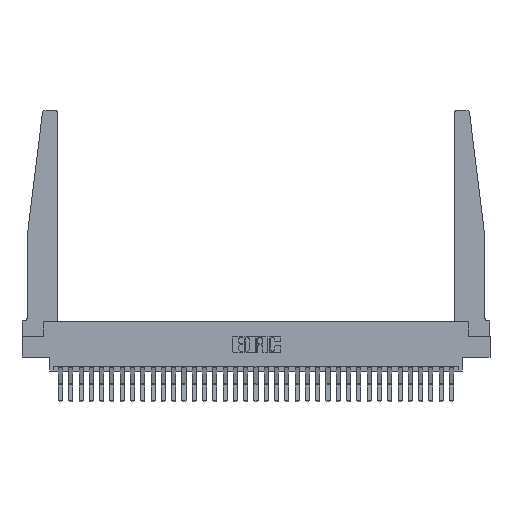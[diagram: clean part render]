
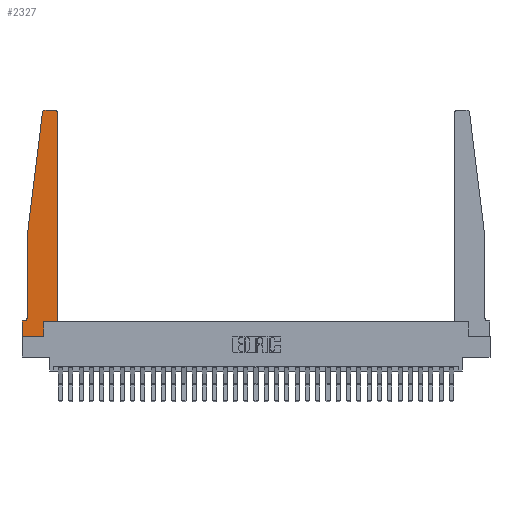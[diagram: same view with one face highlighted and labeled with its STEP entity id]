
A CAD part, top view. The second image highlights one B-rep face of the part: STEP entity #2327.
In plain terms, the highlighted planar face has unit normal (0, 0, 1).
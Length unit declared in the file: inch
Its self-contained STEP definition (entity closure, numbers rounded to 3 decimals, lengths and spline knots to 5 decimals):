
#421 = DIRECTION ( 'NONE',  ( -1., 0., 0. ) ) ;
#681 = VERTEX_POINT ( 'NONE', #3958 ) ;
#983 = VERTEX_POINT ( 'NONE', #4338 ) ;
#1861 = ORIENTED_EDGE ( 'NONE', *, *, #19803, .T. ) ;
#2134 = DIRECTION ( 'NONE',  ( 1., 0., 0. ) ) ;
#2315 = LINE ( 'NONE', #6900, #6386 ) ;
#2326 = ORIENTED_EDGE ( 'NONE', *, *, #6308, .T. ) ;
#2327 = ADVANCED_FACE ( 'NONE', ( #4654 ), #8937, .T. ) ;
#2483 = ORIENTED_EDGE ( 'NONE', *, *, #20605, .T. ) ;
#2792 = VECTOR ( 'NONE', #24482, 39.37008 ) ;
#2905 = VERTEX_POINT ( 'NONE', #14592 ) ;
#3089 = LINE ( 'NONE', #12745, #2792 ) ;
#3877 = VERTEX_POINT ( 'NONE', #20124 ) ;
#3941 = CARTESIAN_POINT ( 'NONE',  ( 0.395, 2.72, 0.37 ) ) ;
#3958 = CARTESIAN_POINT ( 'NONE',  ( 0.395, 2.75, 0.37 ) ) ;
#4250 = CARTESIAN_POINT ( 'NONE',  ( 0.065, 1.25, 0.37 ) ) ;
#4338 = CARTESIAN_POINT ( 'NONE',  ( 0.2605, 0.18, 0.37 ) ) ;
#4415 = ORIENTED_EDGE ( 'NONE', *, *, #16764, .T. ) ;
#4654 = FACE_OUTER_BOUND ( 'NONE', #31258, .T. ) ;
#4717 = VERTEX_POINT ( 'NONE', #27484 ) ;
#4791 = CIRCLE ( 'NONE', #18977, 0.03 ) ;
#5260 = VECTOR ( 'NONE', #11361, 39.37008 ) ;
#5397 = ORIENTED_EDGE ( 'NONE', *, *, #14882, .T. ) ;
#6088 = ORIENTED_EDGE ( 'NONE', *, *, #12064, .T. ) ;
#6089 = VECTOR ( 'NONE', #6155, 39.37008 ) ;
#6155 = DIRECTION ( 'NONE',  ( 0., 1., 0. ) ) ;
#6308 = EDGE_CURVE ( 'NONE', #19038, #23447, #10160, .T. ) ;
#6386 = VECTOR ( 'NONE', #28279, 39.37008 ) ;
#6743 = VERTEX_POINT ( 'NONE', #19764 ) ;
#6900 = CARTESIAN_POINT ( 'NONE',  ( 0.25, 2.75, 0.37 ) ) ;
#7389 = LINE ( 'NONE', #12448, #30969 ) ;
#7442 = CARTESIAN_POINT ( 'NONE',  ( 0.425, 0.18, 0.37 ) ) ;
#7578 = CARTESIAN_POINT ( 'NONE',  ( 0.015, 0.2375, 0.37 ) ) ;
#7744 = DIRECTION ( 'NONE',  ( 1., 0., 0. ) ) ;
#8322 = EDGE_CURVE ( 'NONE', #2905, #19038, #23894, .T. ) ;
#8937 = PLANE ( 'NONE',  #20198 ) ;
#9259 = CARTESIAN_POINT ( 'NONE',  ( 0., 0.1875, 0.37 ) ) ;
#9365 = EDGE_CURVE ( 'NONE', #21525, #983, #3089, .T. ) ;
#9889 = ORIENTED_EDGE ( 'NONE', *, *, #14548, .T. ) ;
#10160 = LINE ( 'NONE', #25352, #28946 ) ;
#11048 = LINE ( 'NONE', #18055, #6089 ) ;
#11361 = DIRECTION ( 'NONE',  ( -0.122, -0.992, 0. ) ) ;
#12064 = EDGE_CURVE ( 'NONE', #4717, #21525, #22014, .T. ) ;
#12083 = CARTESIAN_POINT ( 'NONE',  ( 0.065, 1.25, 0.37 ) ) ;
#12448 = CARTESIAN_POINT ( 'NONE',  ( 0.065, 0.1875, 0.37 ) ) ;
#12745 = CARTESIAN_POINT ( 'NONE',  ( 0.2605, 0.18, 0.37 ) ) ;
#13097 = VECTOR ( 'NONE', #20779, 39.37008 ) ;
#13177 = ORIENTED_EDGE ( 'NONE', *, *, #8322, .T. ) ;
#13376 = CIRCLE ( 'NONE', #22991, 0.03 ) ;
#13601 = DIRECTION ( 'NONE',  ( 0., 0., 1. ) ) ;
#14065 = VERTEX_POINT ( 'NONE', #17497 ) ;
#14548 = EDGE_CURVE ( 'NONE', #21659, #681, #13376, .T. ) ;
#14565 = CARTESIAN_POINT ( 'NONE',  ( 0.27653, 2.72, 0.37 ) ) ;
#14592 = CARTESIAN_POINT ( 'NONE',  ( 0.24675, 2.72367, 0.37 ) ) ;
#14882 = EDGE_CURVE ( 'NONE', #14065, #2905, #4791, .T. ) ;
#15247 = VERTEX_POINT ( 'NONE', #19279 ) ;
#15493 = CARTESIAN_POINT ( 'NONE',  ( 0.2605, 0., 0.37 ) ) ;
#15841 = DIRECTION ( 'NONE',  ( 1., 0., 0. ) ) ;
#16133 = EDGE_CURVE ( 'NONE', #983, #6743, #29144, .T. ) ;
#16400 = VECTOR ( 'NONE', #29135, 39.37008 ) ;
#16764 = EDGE_CURVE ( 'NONE', #681, #14065, #2315, .T. ) ;
#17497 = CARTESIAN_POINT ( 'NONE',  ( 0.27653, 2.75, 0.37 ) ) ;
#17952 = EDGE_CURVE ( 'NONE', #3877, #4717, #18243, .T. ) ;
#18055 = CARTESIAN_POINT ( 'NONE',  ( 0.425, 0.18, 0.37 ) ) ;
#18243 = LINE ( 'NONE', #27896, #13097 ) ;
#18793 = CIRCLE ( 'NONE', #21830, 0.05 ) ;
#18930 = DIRECTION ( 'NONE',  ( 0., 0., 1. ) ) ;
#18977 = AXIS2_PLACEMENT_3D ( 'NONE', #14565, #29446, #7744 ) ;
#19038 = VERTEX_POINT ( 'NONE', #12083 ) ;
#19279 = CARTESIAN_POINT ( 'NONE',  ( 0.015, 0.1875, 0.37 ) ) ;
#19478 = CARTESIAN_POINT ( 'NONE',  ( 0., 0., 0.37 ) ) ;
#19764 = CARTESIAN_POINT ( 'NONE',  ( 0.425, 0.18, 0.37 ) ) ;
#19790 = DIRECTION ( 'NONE',  ( 1., 0., 0. ) ) ;
#19803 = EDGE_CURVE ( 'NONE', #6743, #21659, #11048, .T. ) ;
#20124 = CARTESIAN_POINT ( 'NONE',  ( 0., 0.1875, 0.37 ) ) ;
#20135 = EDGE_CURVE ( 'NONE', #23447, #15247, #18793, .T. ) ;
#20198 = AXIS2_PLACEMENT_3D ( 'NONE', #9259, #18930, #2134 ) ;
#20605 = EDGE_CURVE ( 'NONE', #15247, #3877, #7389, .T. ) ;
#20779 = DIRECTION ( 'NONE',  ( 0., -1., 0. ) ) ;
#21525 = VERTEX_POINT ( 'NONE', #15493 ) ;
#21659 = VERTEX_POINT ( 'NONE', #25890 ) ;
#21830 = AXIS2_PLACEMENT_3D ( 'NONE', #7578, #29435, #21844 ) ;
#21844 = DIRECTION ( 'NONE',  ( -1., 0., 0. ) ) ;
#22014 = LINE ( 'NONE', #19478, #16400 ) ;
#22345 = ORIENTED_EDGE ( 'NONE', *, *, #20135, .T. ) ;
#22824 = DIRECTION ( 'NONE',  ( 0., -1., 0. ) ) ;
#22991 = AXIS2_PLACEMENT_3D ( 'NONE', #3941, #13601, #15841 ) ;
#23447 = VERTEX_POINT ( 'NONE', #24123 ) ;
#23894 = LINE ( 'NONE', #4250, #5260 ) ;
#24123 = CARTESIAN_POINT ( 'NONE',  ( 0.065, 0.2375, 0.37 ) ) ;
#24482 = DIRECTION ( 'NONE',  ( 0., 1., 0. ) ) ;
#25352 = CARTESIAN_POINT ( 'NONE',  ( 0.065, 1.25, 0.37 ) ) ;
#25890 = CARTESIAN_POINT ( 'NONE',  ( 0.425, 2.72, 0.37 ) ) ;
#27230 = ORIENTED_EDGE ( 'NONE', *, *, #16133, .T. ) ;
#27484 = CARTESIAN_POINT ( 'NONE',  ( 0., 0., 0.37 ) ) ;
#27604 = VECTOR ( 'NONE', #19790, 39.37008 ) ;
#27896 = CARTESIAN_POINT ( 'NONE',  ( 0., 0., 0.37 ) ) ;
#28279 = DIRECTION ( 'NONE',  ( -1., 0., 0. ) ) ;
#28532 = ORIENTED_EDGE ( 'NONE', *, *, #9365, .T. ) ;
#28946 = VECTOR ( 'NONE', #22824, 39.37008 ) ;
#29135 = DIRECTION ( 'NONE',  ( 1., 0., 0. ) ) ;
#29144 = LINE ( 'NONE', #7442, #27604 ) ;
#29435 = DIRECTION ( 'NONE',  ( 0., 0., -1. ) ) ;
#29446 = DIRECTION ( 'NONE',  ( 0., 0., 1. ) ) ;
#29686 = ORIENTED_EDGE ( 'NONE', *, *, #17952, .T. ) ;
#30969 = VECTOR ( 'NONE', #421, 39.37008 ) ;
#31258 = EDGE_LOOP ( 'NONE', ( #4415, #5397, #13177, #2326, #22345, #2483, #29686, #6088, #28532, #27230, #1861, #9889 ) ) ;
